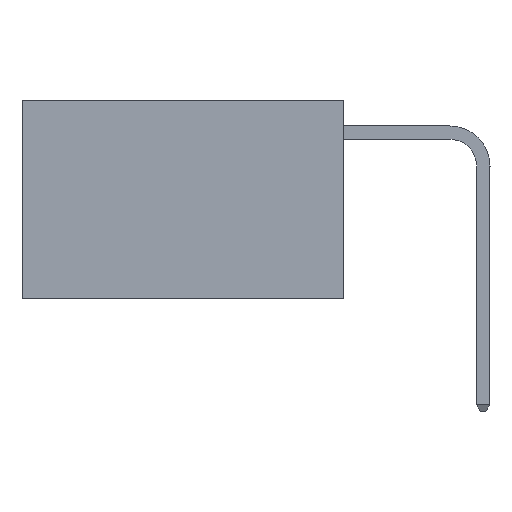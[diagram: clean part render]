
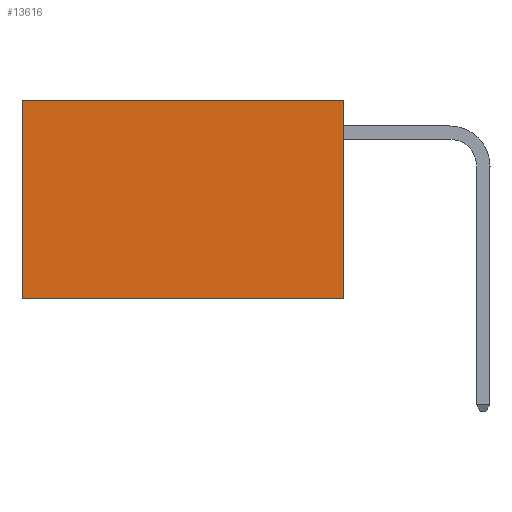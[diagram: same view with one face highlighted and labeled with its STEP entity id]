
A CAD part, left-side view. The second image highlights one B-rep face of the part: STEP entity #13616.
In plain terms, the highlighted planar face has unit normal (-1, 0, 0).
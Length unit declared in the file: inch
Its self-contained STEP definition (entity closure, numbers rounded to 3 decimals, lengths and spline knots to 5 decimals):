
#272 = VECTOR ( 'NONE', #22993, 39.37008 ) ;
#405 = CARTESIAN_POINT ( 'NONE',  ( 0.2625, 0., 0. ) ) ;
#1779 = CARTESIAN_POINT ( 'NONE',  ( 0.2625, 0., 0. ) ) ;
#1818 = ORIENTED_EDGE ( 'NONE', *, *, #9835, .T. ) ;
#2599 = CARTESIAN_POINT ( 'NONE',  ( 0.2625, 0., -0.37 ) ) ;
#3380 = LINE ( 'NONE', #23102, #22249 ) ;
#5312 = LINE ( 'NONE', #17388, #272 ) ;
#5559 = PLANE ( 'NONE',  #12819 ) ;
#5565 = CARTESIAN_POINT ( 'NONE',  ( 0.2625, 0., -0.37 ) ) ;
#5823 = FACE_OUTER_BOUND ( 'NONE', #21416, .T. ) ;
#7474 = DIRECTION ( 'NONE',  ( 1., 0., 0. ) ) ;
#7628 = EDGE_CURVE ( 'NONE', #19978, #11285, #11754, .T. ) ;
#7892 = ORIENTED_EDGE ( 'NONE', *, *, #7628, .F. ) ;
#8274 = CARTESIAN_POINT ( 'NONE',  ( 0.2625, 0.6, -0.37 ) ) ;
#9402 = DIRECTION ( 'NONE',  ( 0., 1., 0. ) ) ;
#9835 = EDGE_CURVE ( 'NONE', #16492, #15836, #22558, .T. ) ;
#9975 = DIRECTION ( 'NONE',  ( 0., 0., -1. ) ) ;
#10051 = EDGE_CURVE ( 'NONE', #15836, #11285, #3380, .T. ) ;
#11017 = ORIENTED_EDGE ( 'NONE', *, *, #10051, .T. ) ;
#11175 = VECTOR ( 'NONE', #11268, 39.37008 ) ;
#11268 = DIRECTION ( 'NONE',  ( 0., 1., 0. ) ) ;
#11285 = VERTEX_POINT ( 'NONE', #8274 ) ;
#11754 = LINE ( 'NONE', #5565, #11175 ) ;
#12819 = AXIS2_PLACEMENT_3D ( 'NONE', #12964, #7474, #20635 ) ;
#12964 = CARTESIAN_POINT ( 'NONE',  ( 0.2625, 0., 0. ) ) ;
#13616 = ADVANCED_FACE ( 'NONE', ( #5823 ), #5559, .F. ) ;
#15836 = VERTEX_POINT ( 'NONE', #23094 ) ;
#16492 = VERTEX_POINT ( 'NONE', #405 ) ;
#17388 = CARTESIAN_POINT ( 'NONE',  ( 0.2625, 0., 0. ) ) ;
#19174 = EDGE_CURVE ( 'NONE', #16492, #19978, #5312, .T. ) ;
#19978 = VERTEX_POINT ( 'NONE', #2599 ) ;
#20635 = DIRECTION ( 'NONE',  ( 0., 0., -1. ) ) ;
#21416 = EDGE_LOOP ( 'NONE', ( #11017, #7892, #23648, #1818 ) ) ;
#21979 = VECTOR ( 'NONE', #9402, 39.37008 ) ;
#22249 = VECTOR ( 'NONE', #9975, 39.37008 ) ;
#22558 = LINE ( 'NONE', #1779, #21979 ) ;
#22993 = DIRECTION ( 'NONE',  ( 0., 0., -1. ) ) ;
#23094 = CARTESIAN_POINT ( 'NONE',  ( 0.2625, 0.6, 0. ) ) ;
#23102 = CARTESIAN_POINT ( 'NONE',  ( 0.2625, 0.6, 0. ) ) ;
#23648 = ORIENTED_EDGE ( 'NONE', *, *, #19174, .F. ) ;
